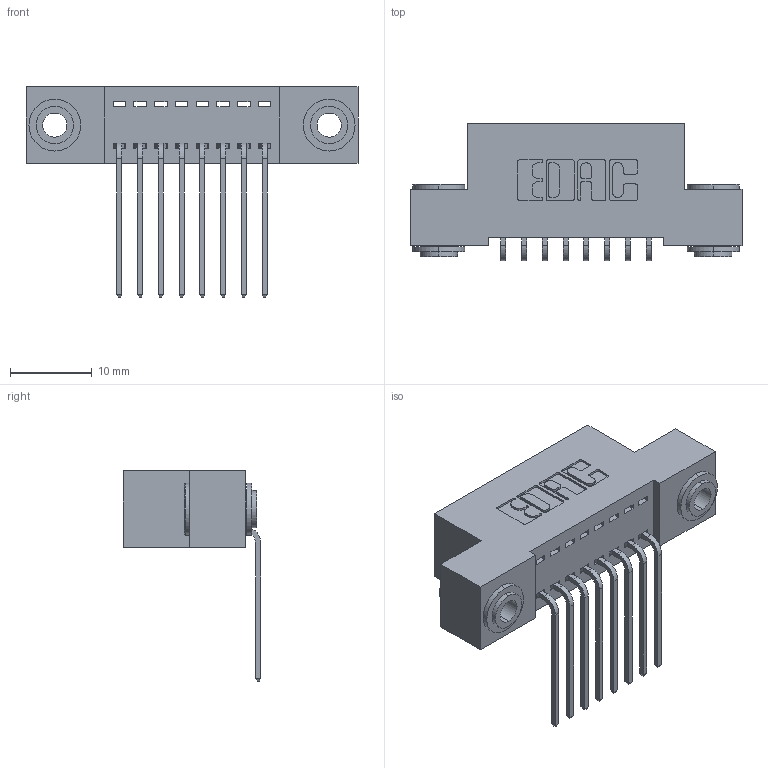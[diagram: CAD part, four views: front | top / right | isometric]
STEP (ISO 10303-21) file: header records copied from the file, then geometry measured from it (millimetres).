
FILE_DESCRIPTION (( 'STEP AP203' ), '1' );
FILE_NAME ('342-008-559-103.STEP', '2019-10-01T13:18:18', ( '' ), ( '' ), 'SwSTEP 2.0', 'SolidWorks 2016', '' );
FILE_SCHEMA (( 'CONFIG_CONTROL_DESIGN' ));
Length unit declared in the file: inch
Products named in the file (4): 345-292-001_558 559 Tail - 1; 342-250-002_345-250-002-102; 342-008-559-103; 342 Part_.156 TH
Assembly tree (11 placements, depth 2):
  342-008-559-103
    342 Part_.156 TH
    345-292-001_558 559 Tail - 1  x8
    342-250-002_345-250-002-102  x2
Bounding box: 40.64 x 16.83 x 25.78 mm (x, y, z)
Volume: 3487.6 mm3; surface area: 4864 mm2
Topology: 11 solids, 11 shells, 628 faces, 1831 edges, 1206 vertices
Faces by surface type: plane 428, cylinder 192, cone 8
Entity records: 9890 total; most frequent: CARTESIAN_POINT 1689, ORIENTED_EDGE 1626, DIRECTION 1527, EDGE_CURVE 813, LINE 661, VECTOR 661, VERTEX_POINT 538, AXIS2_PLACEMENT_3D 433
